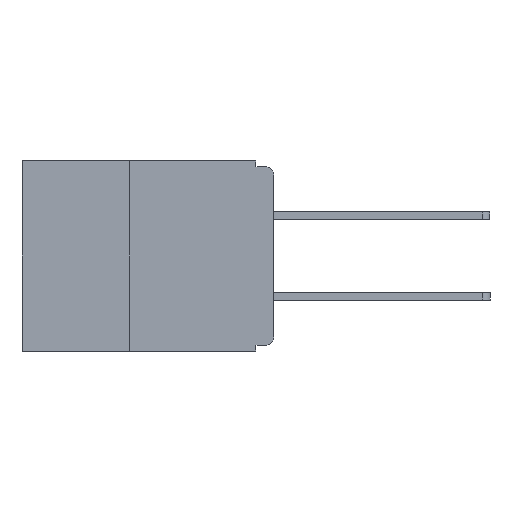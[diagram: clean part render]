
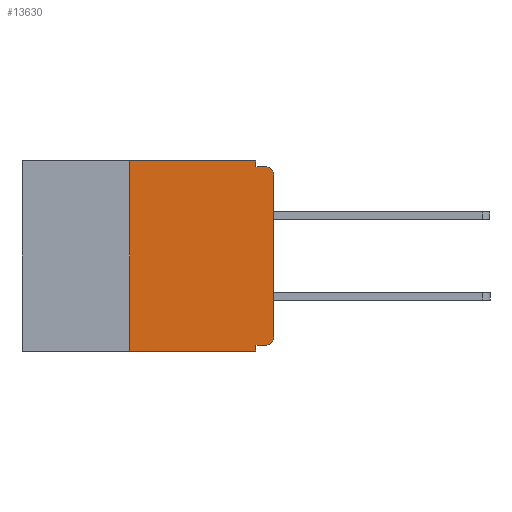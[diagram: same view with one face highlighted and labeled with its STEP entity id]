
A CAD part, left-side view. The second image highlights one B-rep face of the part: STEP entity #13630.
In plain terms, the highlighted planar face has unit normal (-1, 0, 0).
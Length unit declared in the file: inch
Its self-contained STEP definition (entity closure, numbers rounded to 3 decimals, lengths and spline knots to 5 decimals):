
#44 = CARTESIAN_POINT ( 'NONE',  ( 0., 0., -0.32 ) ) ;
#704 = VECTOR ( 'NONE', #14371, 39.37008 ) ;
#1604 = CARTESIAN_POINT ( 'NONE',  ( 0., 0.437, -0.33 ) ) ;
#2120 = CARTESIAN_POINT ( 'NONE',  ( 0., 0.031, -0.33 ) ) ;
#2634 = DIRECTION ( 'NONE',  ( 0., -1., 0. ) ) ;
#2745 = EDGE_CURVE ( 'NONE', #16834, #11799, #6782, .T. ) ;
#2790 = EDGE_CURVE ( 'NONE', #7515, #18115, #21634, .T. ) ;
#2809 = VECTOR ( 'NONE', #11289, 39.37008 ) ;
#2828 = DIRECTION ( 'NONE',  ( -1., 0., 0. ) ) ;
#3089 = VERTEX_POINT ( 'NONE', #10791 ) ;
#3094 = VECTOR ( 'NONE', #14077, 39.37008 ) ;
#3998 = VERTEX_POINT ( 'NONE', #22717 ) ;
#4321 = DIRECTION ( 'NONE',  ( 0., 1., 0. ) ) ;
#4673 = ORIENTED_EDGE ( 'NONE', *, *, #4976, .T. ) ;
#4976 = EDGE_CURVE ( 'NONE', #18943, #12366, #17045, .T. ) ;
#5290 = EDGE_CURVE ( 'NONE', #20074, #3998, #20320, .T. ) ;
#5966 = CARTESIAN_POINT ( 'NONE',  ( 0., 0., -0.01 ) ) ;
#6066 = VECTOR ( 'NONE', #2634, 39.37008 ) ;
#6455 = DIRECTION ( 'NONE',  ( 0., 0., -1. ) ) ;
#6711 = DIRECTION ( 'NONE',  ( 0., 0., -1. ) ) ;
#6782 = LINE ( 'NONE', #26005, #704 ) ;
#7388 = CARTESIAN_POINT ( 'NONE',  ( 0., 0., -0.305 ) ) ;
#7515 = VERTEX_POINT ( 'NONE', #17512 ) ;
#7919 = EDGE_CURVE ( 'NONE', #20074, #16834, #13381, .T. ) ;
#7969 = DIRECTION ( 'NONE',  ( 0., -1., 0. ) ) ;
#8261 = ORIENTED_EDGE ( 'NONE', *, *, #2790, .F. ) ;
#8364 = LINE ( 'NONE', #2120, #3094 ) ;
#8413 = AXIS2_PLACEMENT_3D ( 'NONE', #14742, #2828, #16813 ) ;
#8457 = CARTESIAN_POINT ( 'NONE',  ( 0., 0.031, 0. ) ) ;
#8570 = DIRECTION ( 'NONE',  ( -1., 0., 0. ) ) ;
#9146 = AXIS2_PLACEMENT_3D ( 'NONE', #10629, #18768, #6711 ) ;
#9251 = LINE ( 'NONE', #5966, #24653 ) ;
#9769 = ORIENTED_EDGE ( 'NONE', *, *, #10601, .F. ) ;
#9777 = LINE ( 'NONE', #8457, #25163 ) ;
#9834 = AXIS2_PLACEMENT_3D ( 'NONE', #20743, #8570, #22708 ) ;
#10266 = FACE_OUTER_BOUND ( 'NONE', #19641, .T. ) ;
#10454 = CARTESIAN_POINT ( 'NONE',  ( 0., 0.031, 0. ) ) ;
#10601 = EDGE_CURVE ( 'NONE', #11799, #16416, #9777, .T. ) ;
#10629 = CARTESIAN_POINT ( 'NONE',  ( 0., 0.437, 0. ) ) ;
#10791 = CARTESIAN_POINT ( 'NONE',  ( 0., 0.015, -0.01 ) ) ;
#10909 = ORIENTED_EDGE ( 'NONE', *, *, #25855, .F. ) ;
#11173 = CARTESIAN_POINT ( 'NONE',  ( 0., 0.25, -0.33 ) ) ;
#11289 = DIRECTION ( 'NONE',  ( 0., 0., 1. ) ) ;
#11799 = VERTEX_POINT ( 'NONE', #10454 ) ;
#12366 = VERTEX_POINT ( 'NONE', #18268 ) ;
#12573 = CARTESIAN_POINT ( 'NONE',  ( 0., 0.25, 0. ) ) ;
#12580 = CARTESIAN_POINT ( 'NONE',  ( 0., 0.25, -0.33 ) ) ;
#12622 = PLANE ( 'NONE',  #9146 ) ;
#13252 = ORIENTED_EDGE ( 'NONE', *, *, #24770, .T. ) ;
#13381 = LINE ( 'NONE', #11173, #2809 ) ;
#13630 = ADVANCED_FACE ( 'NONE', ( #10266 ), #12622, .F. ) ;
#14077 = DIRECTION ( 'NONE',  ( 0., 0., -1. ) ) ;
#14371 = DIRECTION ( 'NONE',  ( 0., -1., 0. ) ) ;
#14742 = CARTESIAN_POINT ( 'NONE',  ( 0., 0.015, -0.305 ) ) ;
#14757 = ORIENTED_EDGE ( 'NONE', *, *, #7919, .F. ) ;
#14799 = EDGE_CURVE ( 'NONE', #16416, #3089, #9251, .T. ) ;
#15775 = ORIENTED_EDGE ( 'NONE', *, *, #2745, .F. ) ;
#16416 = VERTEX_POINT ( 'NONE', #17011 ) ;
#16813 = DIRECTION ( 'NONE',  ( 0., 0., -1. ) ) ;
#16834 = VERTEX_POINT ( 'NONE', #12573 ) ;
#16921 = CARTESIAN_POINT ( 'NONE',  ( 0., 0.031, -0.32 ) ) ;
#17011 = CARTESIAN_POINT ( 'NONE',  ( 0., 0.031, -0.01 ) ) ;
#17045 = LINE ( 'NONE', #18911, #21858 ) ;
#17512 = CARTESIAN_POINT ( 'NONE',  ( 0., 0.015, -0.32 ) ) ;
#18115 = VERTEX_POINT ( 'NONE', #16921 ) ;
#18268 = CARTESIAN_POINT ( 'NONE',  ( 0., 0., -0.025 ) ) ;
#18433 = ORIENTED_EDGE ( 'NONE', *, *, #5290, .T. ) ;
#18593 = DIRECTION ( 'NONE',  ( 0., 0., 1. ) ) ;
#18768 = DIRECTION ( 'NONE',  ( 1., 0., 0. ) ) ;
#18911 = CARTESIAN_POINT ( 'NONE',  ( 0., 0., 0. ) ) ;
#18943 = VERTEX_POINT ( 'NONE', #7388 ) ;
#19641 = EDGE_LOOP ( 'NONE', ( #4673, #13252, #22180, #9769, #15775, #14757, #18433, #10909, #8261, #20325 ) ) ;
#20074 = VERTEX_POINT ( 'NONE', #12580 ) ;
#20320 = LINE ( 'NONE', #1604, #6066 ) ;
#20325 = ORIENTED_EDGE ( 'NONE', *, *, #20864, .T. ) ;
#20695 = CIRCLE ( 'NONE', #8413, 0.015 ) ;
#20743 = CARTESIAN_POINT ( 'NONE',  ( 0., 0.015, -0.025 ) ) ;
#20864 = EDGE_CURVE ( 'NONE', #7515, #18943, #20695, .T. ) ;
#21030 = VECTOR ( 'NONE', #4321, 39.37008 ) ;
#21634 = LINE ( 'NONE', #44, #21030 ) ;
#21858 = VECTOR ( 'NONE', #18593, 39.37008 ) ;
#22180 = ORIENTED_EDGE ( 'NONE', *, *, #14799, .F. ) ;
#22708 = DIRECTION ( 'NONE',  ( 0., 0., -1. ) ) ;
#22717 = CARTESIAN_POINT ( 'NONE',  ( 0., 0.031, -0.33 ) ) ;
#24653 = VECTOR ( 'NONE', #7969, 39.37008 ) ;
#24770 = EDGE_CURVE ( 'NONE', #12366, #3089, #24771, .T. ) ;
#24771 = CIRCLE ( 'NONE', #9834, 0.015 ) ;
#25163 = VECTOR ( 'NONE', #6455, 39.37008 ) ;
#25855 = EDGE_CURVE ( 'NONE', #18115, #3998, #8364, .T. ) ;
#26005 = CARTESIAN_POINT ( 'NONE',  ( 0., 0.437, 0. ) ) ;
